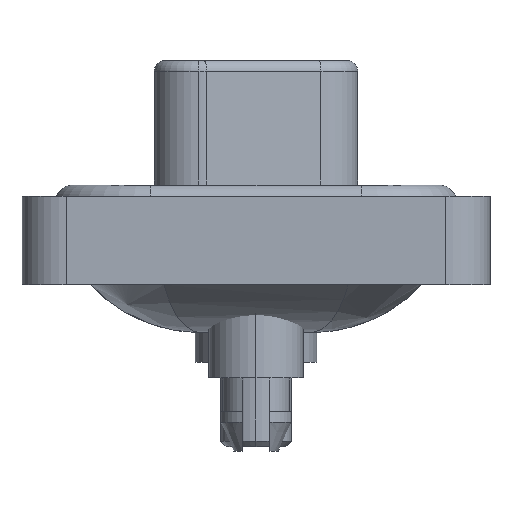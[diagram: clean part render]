
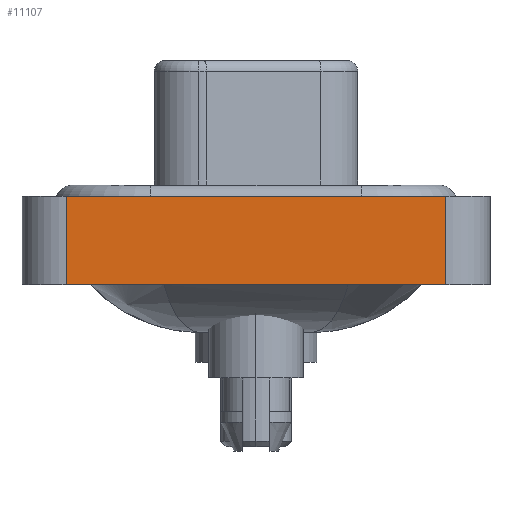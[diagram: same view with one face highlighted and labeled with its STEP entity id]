
A CAD part, left-side view. The second image highlights one B-rep face of the part: STEP entity #11107.
In plain terms, the highlighted planar face has unit normal (-1, 0, 0).
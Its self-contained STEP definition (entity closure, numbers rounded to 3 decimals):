
#425 = EDGE_LOOP ( 'NONE', ( #9469, #2561, #9005, #18735 ) ) ;
#687 = FACE_OUTER_BOUND ( 'NONE', #425, .T. ) ;
#1642 = CARTESIAN_POINT ( 'NONE',  ( -7.3, -8.55, -3.6 ) ) ;
#2561 = ORIENTED_EDGE ( 'NONE', *, *, #6494, .F. ) ;
#4268 = VECTOR ( 'NONE', #10969, 1000. ) ;
#4395 = DIRECTION ( 'NONE',  ( -1., 0., 0. ) ) ;
#4749 = EDGE_CURVE ( 'NONE', #13135, #10663, #13362, .T. ) ;
#5095 = DIRECTION ( 'NONE',  ( 0., 0., 1. ) ) ;
#6494 = EDGE_CURVE ( 'NONE', #20352, #10663, #20960, .T. ) ;
#7226 = CARTESIAN_POINT ( 'NONE',  ( -7.3, 8.55, -3.6 ) ) ;
#8832 = DIRECTION ( 'NONE',  ( 0., 0., 1. ) ) ;
#9005 = ORIENTED_EDGE ( 'NONE', *, *, #15299, .F. ) ;
#9210 = CARTESIAN_POINT ( 'NONE',  ( -7.3, -8.55, 0.4 ) ) ;
#9469 = ORIENTED_EDGE ( 'NONE', *, *, #4749, .T. ) ;
#10663 = VERTEX_POINT ( 'NONE', #19901 ) ;
#10690 = CARTESIAN_POINT ( 'NONE',  ( -7.3, -8.55, -3.6 ) ) ;
#10969 = DIRECTION ( 'NONE',  ( 0., -1., 0. ) ) ;
#11107 = ADVANCED_FACE ( 'NONE', ( #687 ), #19283, .T. ) ;
#11924 = DIRECTION ( 'NONE',  ( 0., 0., 1. ) ) ;
#13135 = VERTEX_POINT ( 'NONE', #1642 ) ;
#13362 = LINE ( 'NONE', #14867, #18956 ) ;
#14867 = CARTESIAN_POINT ( 'NONE',  ( -7.3, -8.55, -3.6 ) ) ;
#15026 = AXIS2_PLACEMENT_3D ( 'NONE', #10690, #4395, #8832 ) ;
#15299 = EDGE_CURVE ( 'NONE', #20582, #20352, #17009, .T. ) ;
#16675 = LINE ( 'NONE', #20045, #16869 ) ;
#16869 = VECTOR ( 'NONE', #18535, 1000. ) ;
#17009 = LINE ( 'NONE', #7226, #18472 ) ;
#18472 = VECTOR ( 'NONE', #11924, 1000. ) ;
#18535 = DIRECTION ( 'NONE',  ( 0., -1., 0. ) ) ;
#18735 = ORIENTED_EDGE ( 'NONE', *, *, #21219, .T. ) ;
#18956 = VECTOR ( 'NONE', #5095, 1000. ) ;
#19283 = PLANE ( 'NONE',  #15026 ) ;
#19901 = CARTESIAN_POINT ( 'NONE',  ( -7.3, -8.55, 0.4 ) ) ;
#20045 = CARTESIAN_POINT ( 'NONE',  ( -7.3, -8.55, -3.6 ) ) ;
#20284 = CARTESIAN_POINT ( 'NONE',  ( -7.3, 8.55, 0.4 ) ) ;
#20352 = VERTEX_POINT ( 'NONE', #20284 ) ;
#20582 = VERTEX_POINT ( 'NONE', #20941 ) ;
#20941 = CARTESIAN_POINT ( 'NONE',  ( -7.3, 8.55, -3.6 ) ) ;
#20960 = LINE ( 'NONE', #9210, #4268 ) ;
#21219 = EDGE_CURVE ( 'NONE', #20582, #13135, #16675, .T. ) ;
